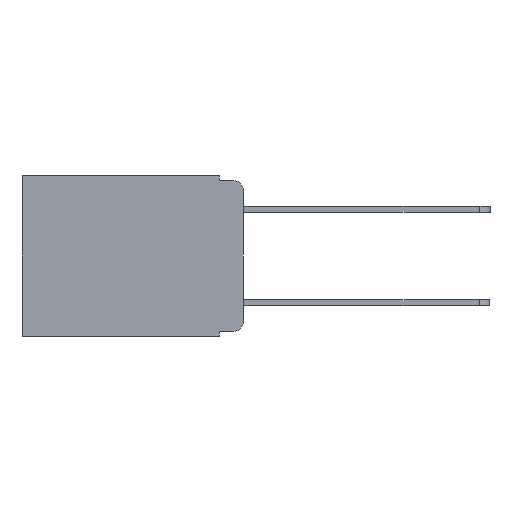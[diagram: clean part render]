
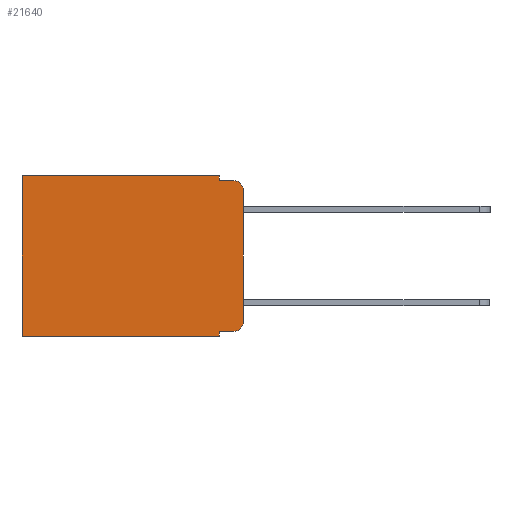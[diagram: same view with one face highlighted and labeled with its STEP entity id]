
A CAD part, left-side view. The second image highlights one B-rep face of the part: STEP entity #21640.
In plain terms, the highlighted planar face has unit normal (-1, 0, 0).
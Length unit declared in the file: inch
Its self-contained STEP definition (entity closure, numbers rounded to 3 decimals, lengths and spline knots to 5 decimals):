
#1018 = ORIENTED_EDGE ( 'NONE', *, *, #13538, .F. ) ;
#1898 = VERTEX_POINT ( 'NONE', #6375 ) ;
#2039 = DIRECTION ( 'NONE',  ( 0., -1., 0. ) ) ;
#2262 = ORIENTED_EDGE ( 'NONE', *, *, #17249, .T. ) ;
#2439 = CARTESIAN_POINT ( 'NONE',  ( 0.298, 0., -0.343 ) ) ;
#3703 = AXIS2_PLACEMENT_3D ( 'NONE', #18512, #7390, #20271 ) ;
#3705 = VECTOR ( 'NONE', #6809, 39.37008 ) ;
#3727 = DIRECTION ( 'NONE',  ( 0., 0., -1. ) ) ;
#4087 = CARTESIAN_POINT ( 'NONE',  ( 0.298, 0.051, 0. ) ) ;
#4332 = LINE ( 'NONE', #23691, #23311 ) ;
#4413 = DIRECTION ( 'NONE',  ( 0., 1., 0. ) ) ;
#4565 = VERTEX_POINT ( 'NONE', #12594 ) ;
#4600 = VERTEX_POINT ( 'NONE', #18188 ) ;
#4933 = EDGE_CURVE ( 'NONE', #4565, #5252, #9688, .T. ) ;
#5021 = ORIENTED_EDGE ( 'NONE', *, *, #9750, .F. ) ;
#5056 = CARTESIAN_POINT ( 'NONE',  ( 0.298, 0., 0. ) ) ;
#5239 = CARTESIAN_POINT ( 'NONE',  ( 0.298, 0.051, -0.343 ) ) ;
#5252 = VERTEX_POINT ( 'NONE', #20007 ) ;
#5573 = FACE_OUTER_BOUND ( 'NONE', #21685, .T. ) ;
#5631 = VERTEX_POINT ( 'NONE', #21292 ) ;
#5988 = ORIENTED_EDGE ( 'NONE', *, *, #23807, .T. ) ;
#6089 = DIRECTION ( 'NONE',  ( 0., 1., 0. ) ) ;
#6297 = AXIS2_PLACEMENT_3D ( 'NONE', #5056, #18166, #7025 ) ;
#6375 = CARTESIAN_POINT ( 'NONE',  ( 0.298, 0.02, -0.01 ) ) ;
#6503 = AXIS2_PLACEMENT_3D ( 'NONE', #19939, #8944, #21693 ) ;
#6560 = VERTEX_POINT ( 'NONE', #5239 ) ;
#6809 = DIRECTION ( 'NONE',  ( 0., 0., -1. ) ) ;
#6953 = CIRCLE ( 'NONE', #3703, 0.02 ) ;
#7025 = DIRECTION ( 'NONE',  ( 0., 0., -1. ) ) ;
#7098 = VERTEX_POINT ( 'NONE', #14534 ) ;
#7311 = CARTESIAN_POINT ( 'NONE',  ( 0.298, 0., -0.313 ) ) ;
#7390 = DIRECTION ( 'NONE',  ( -1., 0., 0. ) ) ;
#7641 = LINE ( 'NONE', #22182, #21678 ) ;
#8017 = EDGE_CURVE ( 'NONE', #4600, #5631, #13981, .T. ) ;
#8532 = VERTEX_POINT ( 'NONE', #20281 ) ;
#8859 = LINE ( 'NONE', #14343, #3705 ) ;
#8944 = DIRECTION ( 'NONE',  ( -1., 0., 0. ) ) ;
#9065 = LINE ( 'NONE', #2439, #18314 ) ;
#9688 = LINE ( 'NONE', #11761, #18913 ) ;
#9750 = EDGE_CURVE ( 'NONE', #8532, #1898, #4332, .T. ) ;
#10064 = CIRCLE ( 'NONE', #6503, 0.02 ) ;
#10135 = ORIENTED_EDGE ( 'NONE', *, *, #4933, .T. ) ;
#10468 = VERTEX_POINT ( 'NONE', #21189 ) ;
#10751 = ORIENTED_EDGE ( 'NONE', *, *, #23516, .F. ) ;
#11342 = ORIENTED_EDGE ( 'NONE', *, *, #13086, .T. ) ;
#11572 = EDGE_CURVE ( 'NONE', #7098, #23803, #23623, .T. ) ;
#11761 = CARTESIAN_POINT ( 'NONE',  ( 0.298, 0., 0. ) ) ;
#12594 = CARTESIAN_POINT ( 'NONE',  ( 0.298, 0.051, 0. ) ) ;
#13086 = EDGE_CURVE ( 'NONE', #5631, #23803, #10064, .T. ) ;
#13538 = EDGE_CURVE ( 'NONE', #4565, #8532, #8859, .T. ) ;
#13606 = CARTESIAN_POINT ( 'NONE',  ( 0.298, 0., 0. ) ) ;
#13981 = LINE ( 'NONE', #15332, #22351 ) ;
#14243 = VECTOR ( 'NONE', #15480, 39.37008 ) ;
#14343 = CARTESIAN_POINT ( 'NONE',  ( 0.298, 0.051, 0. ) ) ;
#14534 = CARTESIAN_POINT ( 'NONE',  ( 0.298, 0., -0.03 ) ) ;
#14946 = VECTOR ( 'NONE', #22557, 39.37008 ) ;
#15019 = DIRECTION ( 'NONE',  ( 0., -1., 0. ) ) ;
#15296 = EDGE_CURVE ( 'NONE', #4600, #6560, #20247, .T. ) ;
#15332 = CARTESIAN_POINT ( 'NONE',  ( 0.298, 0.051, -0.333 ) ) ;
#15480 = DIRECTION ( 'NONE',  ( 0., 0., -1. ) ) ;
#17249 = EDGE_CURVE ( 'NONE', #5252, #10468, #7641, .T. ) ;
#17403 = ORIENTED_EDGE ( 'NONE', *, *, #8017, .T. ) ;
#18166 = DIRECTION ( 'NONE',  ( 1., 0., 0. ) ) ;
#18188 = CARTESIAN_POINT ( 'NONE',  ( 0.298, 0.051, -0.333 ) ) ;
#18314 = VECTOR ( 'NONE', #4413, 39.37008 ) ;
#18512 = CARTESIAN_POINT ( 'NONE',  ( 0.298, 0.02, -0.03 ) ) ;
#18913 = VECTOR ( 'NONE', #6089, 39.37008 ) ;
#19333 = ORIENTED_EDGE ( 'NONE', *, *, #11572, .F. ) ;
#19939 = CARTESIAN_POINT ( 'NONE',  ( 0.298, 0.02, -0.313 ) ) ;
#20007 = CARTESIAN_POINT ( 'NONE',  ( 0.298, 0.473, 0. ) ) ;
#20247 = LINE ( 'NONE', #4087, #14946 ) ;
#20271 = DIRECTION ( 'NONE',  ( 0., 0., -1. ) ) ;
#20281 = CARTESIAN_POINT ( 'NONE',  ( 0.298, 0.051, -0.01 ) ) ;
#20420 = ORIENTED_EDGE ( 'NONE', *, *, #15296, .F. ) ;
#21189 = CARTESIAN_POINT ( 'NONE',  ( 0.298, 0.473, -0.343 ) ) ;
#21292 = CARTESIAN_POINT ( 'NONE',  ( 0.298, 0.02, -0.333 ) ) ;
#21640 = ADVANCED_FACE ( 'NONE', ( #5573 ), #23321, .F. ) ;
#21678 = VECTOR ( 'NONE', #3727, 39.37008 ) ;
#21685 = EDGE_LOOP ( 'NONE', ( #19333, #5988, #5021, #1018, #10135, #2262, #10751, #20420, #17403, #11342 ) ) ;
#21693 = DIRECTION ( 'NONE',  ( 0., 0., -1. ) ) ;
#22182 = CARTESIAN_POINT ( 'NONE',  ( 0.298, 0.473, 0. ) ) ;
#22351 = VECTOR ( 'NONE', #2039, 39.37008 ) ;
#22557 = DIRECTION ( 'NONE',  ( 0., 0., -1. ) ) ;
#23311 = VECTOR ( 'NONE', #15019, 39.37008 ) ;
#23321 = PLANE ( 'NONE',  #6297 ) ;
#23516 = EDGE_CURVE ( 'NONE', #6560, #10468, #9065, .T. ) ;
#23623 = LINE ( 'NONE', #13606, #14243 ) ;
#23691 = CARTESIAN_POINT ( 'NONE',  ( 0.298, 0.051, -0.01 ) ) ;
#23803 = VERTEX_POINT ( 'NONE', #7311 ) ;
#23807 = EDGE_CURVE ( 'NONE', #7098, #1898, #6953, .T. ) ;
